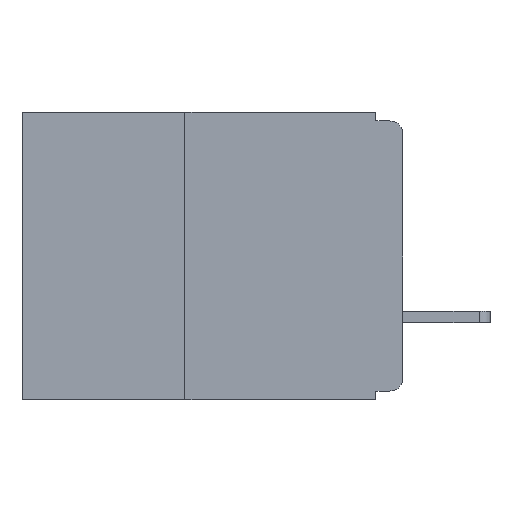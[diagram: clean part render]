
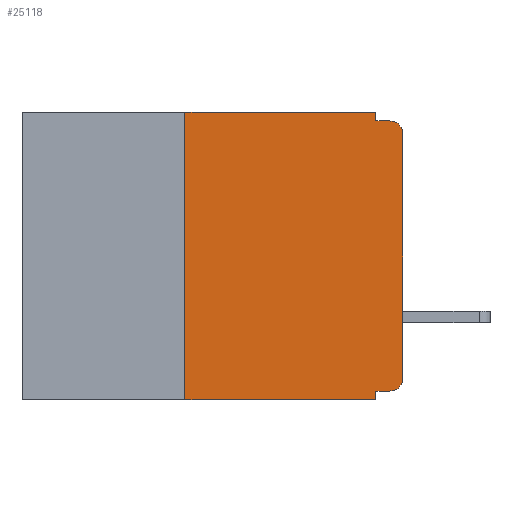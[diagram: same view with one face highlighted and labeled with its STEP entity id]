
A CAD part, left-side view. The second image highlights one B-rep face of the part: STEP entity #25118.
In plain terms, the highlighted planar face has unit normal (-1, 0, 0).
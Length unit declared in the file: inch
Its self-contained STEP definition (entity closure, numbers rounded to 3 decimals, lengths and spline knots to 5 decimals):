
#409 = EDGE_CURVE ( 'NONE', #2121, #1716, #8651, .T. ) ;
#561 = DIRECTION ( 'NONE',  ( -1., 0., 0. ) ) ;
#861 = CIRCLE ( 'NONE', #4283, 0.015 ) ;
#884 = VERTEX_POINT ( 'NONE', #7412 ) ;
#1072 = FACE_OUTER_BOUND ( 'NONE', #9626, .T. ) ;
#1716 = VERTEX_POINT ( 'NONE', #26232 ) ;
#1909 = ORIENTED_EDGE ( 'NONE', *, *, #409, .T. ) ;
#2121 = VERTEX_POINT ( 'NONE', #18477 ) ;
#2167 = CARTESIAN_POINT ( 'NONE',  ( 0., 0.015, -0.025 ) ) ;
#2588 = CIRCLE ( 'NONE', #26084, 0.015 ) ;
#3365 = LINE ( 'NONE', #6337, #14198 ) ;
#3545 = VERTEX_POINT ( 'NONE', #20130 ) ;
#4148 = CARTESIAN_POINT ( 'NONE',  ( 0., 0.437, 0. ) ) ;
#4243 = DIRECTION ( 'NONE',  ( 0., 0., -1. ) ) ;
#4283 = AXIS2_PLACEMENT_3D ( 'NONE', #13575, #561, #15727 ) ;
#4354 = DIRECTION ( 'NONE',  ( 0., 0., -1. ) ) ;
#4821 = CARTESIAN_POINT ( 'NONE',  ( 0., 0., -0.32 ) ) ;
#4879 = VECTOR ( 'NONE', #15771, 39.37008 ) ;
#4990 = CARTESIAN_POINT ( 'NONE',  ( 0., 0.031, 0. ) ) ;
#5932 = VECTOR ( 'NONE', #12976, 39.37008 ) ;
#6325 = VERTEX_POINT ( 'NONE', #8877 ) ;
#6337 = CARTESIAN_POINT ( 'NONE',  ( 0., 0.437, 0. ) ) ;
#6354 = CARTESIAN_POINT ( 'NONE',  ( 0., 0.25, -0.33 ) ) ;
#6534 = EDGE_CURVE ( 'NONE', #11139, #884, #9933, .T. ) ;
#7412 = CARTESIAN_POINT ( 'NONE',  ( 0., 0.015, -0.01 ) ) ;
#8651 = LINE ( 'NONE', #10172, #19433 ) ;
#8699 = ORIENTED_EDGE ( 'NONE', *, *, #11497, .F. ) ;
#8877 = CARTESIAN_POINT ( 'NONE',  ( 0., 0., -0.305 ) ) ;
#9626 = EDGE_LOOP ( 'NONE', ( #15549, #15693, #14159, #15007, #10083, #20979, #1909, #8699, #12950, #10020 ) ) ;
#9933 = LINE ( 'NONE', #13950, #26210 ) ;
#10020 = ORIENTED_EDGE ( 'NONE', *, *, #10260, .T. ) ;
#10083 = ORIENTED_EDGE ( 'NONE', *, *, #21243, .F. ) ;
#10172 = CARTESIAN_POINT ( 'NONE',  ( 0., 0.437, -0.33 ) ) ;
#10260 = EDGE_CURVE ( 'NONE', #26030, #6325, #861, .T. ) ;
#10723 = EDGE_CURVE ( 'NONE', #6325, #17986, #22388, .T. ) ;
#11139 = VERTEX_POINT ( 'NONE', #21282 ) ;
#11375 = CARTESIAN_POINT ( 'NONE',  ( 0., 0.015, -0.32 ) ) ;
#11497 = EDGE_CURVE ( 'NONE', #24250, #1716, #24958, .T. ) ;
#11993 = CARTESIAN_POINT ( 'NONE',  ( 0., 0.25, 0. ) ) ;
#12037 = CARTESIAN_POINT ( 'NONE',  ( 0., 0.031, -0.32 ) ) ;
#12857 = PLANE ( 'NONE',  #19148 ) ;
#12950 = ORIENTED_EDGE ( 'NONE', *, *, #14655, .F. ) ;
#12976 = DIRECTION ( 'NONE',  ( 0., 0., 1. ) ) ;
#13492 = DIRECTION ( 'NONE',  ( 0., -1., 0. ) ) ;
#13575 = CARTESIAN_POINT ( 'NONE',  ( 0., 0.015, -0.305 ) ) ;
#13950 = CARTESIAN_POINT ( 'NONE',  ( 0., 0., -0.01 ) ) ;
#14159 = ORIENTED_EDGE ( 'NONE', *, *, #6534, .F. ) ;
#14198 = VECTOR ( 'NONE', #21391, 39.37008 ) ;
#14537 = VECTOR ( 'NONE', #19917, 39.37008 ) ;
#14655 = EDGE_CURVE ( 'NONE', #26030, #24250, #19574, .T. ) ;
#15007 = ORIENTED_EDGE ( 'NONE', *, *, #19800, .F. ) ;
#15549 = ORIENTED_EDGE ( 'NONE', *, *, #10723, .T. ) ;
#15693 = ORIENTED_EDGE ( 'NONE', *, *, #22981, .T. ) ;
#15727 = DIRECTION ( 'NONE',  ( 0., 0., -1. ) ) ;
#15771 = DIRECTION ( 'NONE',  ( 0., 0., -1. ) ) ;
#16045 = DIRECTION ( 'NONE',  ( 0., 0., -1. ) ) ;
#17173 = DIRECTION ( 'NONE',  ( 1., 0., 0. ) ) ;
#17210 = DIRECTION ( 'NONE',  ( 0., 0., 1. ) ) ;
#17289 = DIRECTION ( 'NONE',  ( -1., 0., 0. ) ) ;
#17828 = CARTESIAN_POINT ( 'NONE',  ( 0., 0., -0.025 ) ) ;
#17986 = VERTEX_POINT ( 'NONE', #17828 ) ;
#18030 = VECTOR ( 'NONE', #17210, 39.37008 ) ;
#18477 = CARTESIAN_POINT ( 'NONE',  ( 0., 0.25, -0.33 ) ) ;
#18717 = LINE ( 'NONE', #6354, #18030 ) ;
#19148 = AXIS2_PLACEMENT_3D ( 'NONE', #4148, #17173, #4243 ) ;
#19433 = VECTOR ( 'NONE', #13492, 39.37008 ) ;
#19574 = LINE ( 'NONE', #4821, #14537 ) ;
#19800 = EDGE_CURVE ( 'NONE', #3545, #11139, #21393, .T. ) ;
#19917 = DIRECTION ( 'NONE',  ( 0., 1., 0. ) ) ;
#20130 = CARTESIAN_POINT ( 'NONE',  ( 0., 0.031, 0. ) ) ;
#20414 = DIRECTION ( 'NONE',  ( 0., -1., 0. ) ) ;
#20979 = ORIENTED_EDGE ( 'NONE', *, *, #24513, .F. ) ;
#21243 = EDGE_CURVE ( 'NONE', #23152, #3545, #3365, .T. ) ;
#21282 = CARTESIAN_POINT ( 'NONE',  ( 0., 0.031, -0.01 ) ) ;
#21391 = DIRECTION ( 'NONE',  ( 0., -1., 0. ) ) ;
#21393 = LINE ( 'NONE', #4990, #4879 ) ;
#22388 = LINE ( 'NONE', #23578, #5932 ) ;
#22981 = EDGE_CURVE ( 'NONE', #17986, #884, #2588, .T. ) ;
#23152 = VERTEX_POINT ( 'NONE', #11993 ) ;
#23578 = CARTESIAN_POINT ( 'NONE',  ( 0., 0., 0. ) ) ;
#24250 = VERTEX_POINT ( 'NONE', #12037 ) ;
#24315 = VECTOR ( 'NONE', #16045, 39.37008 ) ;
#24513 = EDGE_CURVE ( 'NONE', #2121, #23152, #18717, .T. ) ;
#24537 = CARTESIAN_POINT ( 'NONE',  ( 0., 0.031, -0.33 ) ) ;
#24958 = LINE ( 'NONE', #24537, #24315 ) ;
#25118 = ADVANCED_FACE ( 'NONE', ( #1072 ), #12857, .F. ) ;
#26030 = VERTEX_POINT ( 'NONE', #11375 ) ;
#26084 = AXIS2_PLACEMENT_3D ( 'NONE', #2167, #17289, #4354 ) ;
#26210 = VECTOR ( 'NONE', #20414, 39.37008 ) ;
#26232 = CARTESIAN_POINT ( 'NONE',  ( 0., 0.031, -0.33 ) ) ;
